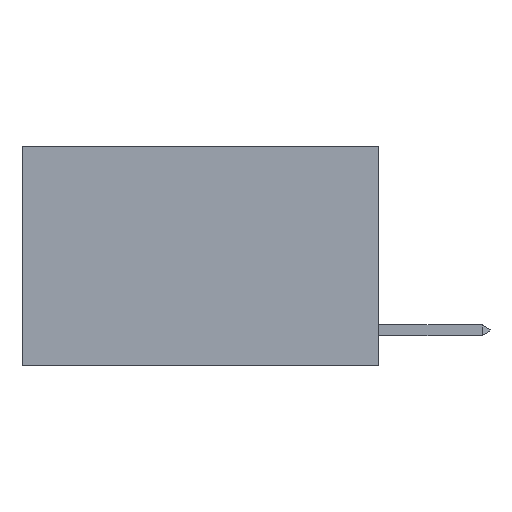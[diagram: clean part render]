
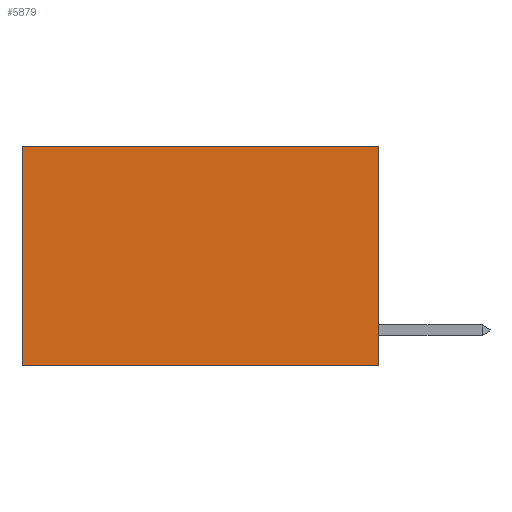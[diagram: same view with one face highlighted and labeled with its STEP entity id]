
A CAD part, left-side view. The second image highlights one B-rep face of the part: STEP entity #5879.
In plain terms, the highlighted planar face has unit normal (-1, 0, 0).
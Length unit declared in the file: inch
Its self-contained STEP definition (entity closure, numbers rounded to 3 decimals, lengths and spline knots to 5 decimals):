
#70 = VERTEX_POINT ( 'NONE', #4512 ) ;
#708 = LINE ( 'NONE', #11198, #1054 ) ;
#866 = DIRECTION ( 'NONE',  ( 0., 0., -1. ) ) ;
#1054 = VECTOR ( 'NONE', #1516, 39.37008 ) ;
#1421 = EDGE_CURVE ( 'NONE', #6769, #70, #6962, .T. ) ;
#1516 = DIRECTION ( 'NONE',  ( 0., 1., 0. ) ) ;
#1816 = ORIENTED_EDGE ( 'NONE', *, *, #1421, .F. ) ;
#1951 = CARTESIAN_POINT ( 'NONE',  ( 0.2625, 0., 0. ) ) ;
#2009 = CARTESIAN_POINT ( 'NONE',  ( 0.2625, 0.6, 0. ) ) ;
#2040 = CARTESIAN_POINT ( 'NONE',  ( 0.2625, 0., 0. ) ) ;
#2614 = DIRECTION ( 'NONE',  ( 0., 0., -1. ) ) ;
#2738 = EDGE_LOOP ( 'NONE', ( #10818, #6543, #1816, #6409 ) ) ;
#2821 = EDGE_CURVE ( 'NONE', #6769, #7012, #4615, .T. ) ;
#2948 = AXIS2_PLACEMENT_3D ( 'NONE', #3715, #7213, #866 ) ;
#3485 = FACE_OUTER_BOUND ( 'NONE', #2738, .T. ) ;
#3715 = CARTESIAN_POINT ( 'NONE',  ( 0.2625, 0., 0. ) ) ;
#4512 = CARTESIAN_POINT ( 'NONE',  ( 0.2625, 0., -0.37 ) ) ;
#4615 = LINE ( 'NONE', #1951, #10280 ) ;
#4741 = VECTOR ( 'NONE', #2614, 39.37008 ) ;
#4920 = VECTOR ( 'NONE', #6337, 39.37008 ) ;
#5876 = EDGE_CURVE ( 'NONE', #7012, #10133, #8019, .T. ) ;
#5879 = ADVANCED_FACE ( 'NONE', ( #3485 ), #8870, .F. ) ;
#6337 = DIRECTION ( 'NONE',  ( 0., 0., -1. ) ) ;
#6409 = ORIENTED_EDGE ( 'NONE', *, *, #2821, .T. ) ;
#6543 = ORIENTED_EDGE ( 'NONE', *, *, #8406, .F. ) ;
#6769 = VERTEX_POINT ( 'NONE', #2040 ) ;
#6962 = LINE ( 'NONE', #10485, #4741 ) ;
#7012 = VERTEX_POINT ( 'NONE', #7595 ) ;
#7213 = DIRECTION ( 'NONE',  ( 1., 0., 0. ) ) ;
#7595 = CARTESIAN_POINT ( 'NONE',  ( 0.2625, 0.6, 0. ) ) ;
#8016 = DIRECTION ( 'NONE',  ( 0., 1., 0. ) ) ;
#8019 = LINE ( 'NONE', #2009, #4920 ) ;
#8207 = CARTESIAN_POINT ( 'NONE',  ( 0.2625, 0.6, -0.37 ) ) ;
#8406 = EDGE_CURVE ( 'NONE', #70, #10133, #708, .T. ) ;
#8870 = PLANE ( 'NONE',  #2948 ) ;
#10133 = VERTEX_POINT ( 'NONE', #8207 ) ;
#10280 = VECTOR ( 'NONE', #8016, 39.37008 ) ;
#10485 = CARTESIAN_POINT ( 'NONE',  ( 0.2625, 0., 0. ) ) ;
#10818 = ORIENTED_EDGE ( 'NONE', *, *, #5876, .T. ) ;
#11198 = CARTESIAN_POINT ( 'NONE',  ( 0.2625, 0., -0.37 ) ) ;
